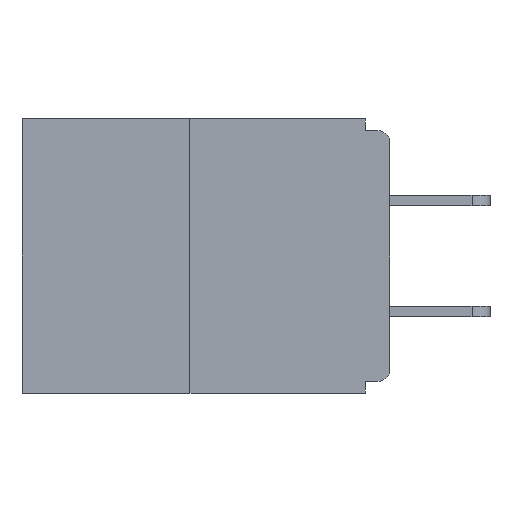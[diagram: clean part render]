
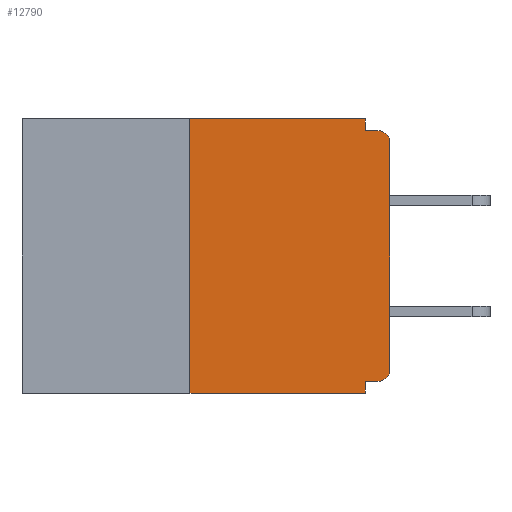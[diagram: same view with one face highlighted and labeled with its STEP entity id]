
A CAD part, left-side view. The second image highlights one B-rep face of the part: STEP entity #12790.
In plain terms, the highlighted planar face has unit normal (-1, 0, 0).
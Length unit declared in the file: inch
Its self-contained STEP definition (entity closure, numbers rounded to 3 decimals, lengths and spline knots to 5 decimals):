
#54 = VECTOR ( 'NONE', #16670, 39.37008 ) ;
#534 = VECTOR ( 'NONE', #2295, 39.37008 ) ;
#1168 = CARTESIAN_POINT ( 'NONE',  ( 0., 0.031, -0.343 ) ) ;
#1472 = CARTESIAN_POINT ( 'NONE',  ( 0., 0.46, 0. ) ) ;
#1593 = DIRECTION ( 'NONE',  ( 0., 0., -1. ) ) ;
#1607 = ORIENTED_EDGE ( 'NONE', *, *, #25234, .F. ) ;
#1665 = LINE ( 'NONE', #11369, #534 ) ;
#2192 = ORIENTED_EDGE ( 'NONE', *, *, #21940, .F. ) ;
#2295 = DIRECTION ( 'NONE',  ( 0., -1., 0. ) ) ;
#2840 = DIRECTION ( 'NONE',  ( 0., 0., -1. ) ) ;
#3822 = CARTESIAN_POINT ( 'NONE',  ( 0., 0.25, 0. ) ) ;
#4606 = EDGE_CURVE ( 'NONE', #22993, #29356, #28138, .T. ) ;
#4746 = CARTESIAN_POINT ( 'NONE',  ( 0., 0.015, -0.313 ) ) ;
#4749 = VERTEX_POINT ( 'NONE', #10541 ) ;
#4824 = CARTESIAN_POINT ( 'NONE',  ( 0., 0., -0.03 ) ) ;
#4848 = VECTOR ( 'NONE', #27370, 39.37008 ) ;
#4927 = CARTESIAN_POINT ( 'NONE',  ( 0., 0.031, 0. ) ) ;
#5744 = ORIENTED_EDGE ( 'NONE', *, *, #18024, .T. ) ;
#6052 = PLANE ( 'NONE',  #17828 ) ;
#6972 = EDGE_CURVE ( 'NONE', #29356, #10993, #19024, .T. ) ;
#7485 = CARTESIAN_POINT ( 'NONE',  ( 0., 0.25, 0. ) ) ;
#7490 = ORIENTED_EDGE ( 'NONE', *, *, #10183, .T. ) ;
#7492 = CIRCLE ( 'NONE', #15079, 0.015 ) ;
#7912 = VERTEX_POINT ( 'NONE', #4824 ) ;
#7968 = VERTEX_POINT ( 'NONE', #7485 ) ;
#8886 = LINE ( 'NONE', #9235, #4848 ) ;
#8995 = AXIS2_PLACEMENT_3D ( 'NONE', #4746, #16107, #18436 ) ;
#9235 = CARTESIAN_POINT ( 'NONE',  ( 0., 0., 0. ) ) ;
#9342 = CARTESIAN_POINT ( 'NONE',  ( 0., 0.46, -0.343 ) ) ;
#9534 = DIRECTION ( 'NONE',  ( 0., -1., 0. ) ) ;
#10183 = EDGE_CURVE ( 'NONE', #7912, #10993, #7492, .T. ) ;
#10427 = DIRECTION ( 'NONE',  ( 0., -1., 0. ) ) ;
#10441 = LINE ( 'NONE', #9342, #25332 ) ;
#10483 = EDGE_CURVE ( 'NONE', #15209, #23033, #10441, .T. ) ;
#10541 = CARTESIAN_POINT ( 'NONE',  ( 0., 0.031, -0.328 ) ) ;
#10993 = VERTEX_POINT ( 'NONE', #16839 ) ;
#11369 = CARTESIAN_POINT ( 'NONE',  ( 0., 0.46, 0. ) ) ;
#11715 = ORIENTED_EDGE ( 'NONE', *, *, #20308, .F. ) ;
#11985 = CARTESIAN_POINT ( 'NONE',  ( 0., 0., -0.015 ) ) ;
#12378 = CARTESIAN_POINT ( 'NONE',  ( 0., 0.25, -0.343 ) ) ;
#12790 = ADVANCED_FACE ( 'NONE', ( #25566 ), #6052, .F. ) ;
#13794 = EDGE_CURVE ( 'NONE', #14344, #4749, #19352, .T. ) ;
#14111 = ORIENTED_EDGE ( 'NONE', *, *, #13794, .F. ) ;
#14344 = VERTEX_POINT ( 'NONE', #16076 ) ;
#15079 = AXIS2_PLACEMENT_3D ( 'NONE', #19094, #26093, #28530 ) ;
#15209 = VERTEX_POINT ( 'NONE', #12378 ) ;
#15305 = EDGE_LOOP ( 'NONE', ( #1607, #2192, #17793, #11715, #14111, #20215, #5744, #7490, #19485, #23784 ) ) ;
#16076 = CARTESIAN_POINT ( 'NONE',  ( 0., 0.015, -0.328 ) ) ;
#16107 = DIRECTION ( 'NONE',  ( -1., 0., 0. ) ) ;
#16670 = DIRECTION ( 'NONE',  ( 0., 0., -1. ) ) ;
#16839 = CARTESIAN_POINT ( 'NONE',  ( 0., 0.015, -0.015 ) ) ;
#16974 = CARTESIAN_POINT ( 'NONE',  ( 0., 0.031, 0. ) ) ;
#17793 = ORIENTED_EDGE ( 'NONE', *, *, #10483, .T. ) ;
#17804 = VERTEX_POINT ( 'NONE', #23931 ) ;
#17828 = AXIS2_PLACEMENT_3D ( 'NONE', #1472, #27124, #1593 ) ;
#18024 = EDGE_CURVE ( 'NONE', #17804, #7912, #8886, .T. ) ;
#18436 = DIRECTION ( 'NONE',  ( 0., 0., -1. ) ) ;
#18606 = VECTOR ( 'NONE', #25016, 39.37008 ) ;
#19024 = LINE ( 'NONE', #11985, #19764 ) ;
#19094 = CARTESIAN_POINT ( 'NONE',  ( 0., 0.015, -0.03 ) ) ;
#19352 = LINE ( 'NONE', #22488, #18606 ) ;
#19485 = ORIENTED_EDGE ( 'NONE', *, *, #6972, .F. ) ;
#19764 = VECTOR ( 'NONE', #9534, 39.37008 ) ;
#20215 = ORIENTED_EDGE ( 'NONE', *, *, #20249, .T. ) ;
#20249 = EDGE_CURVE ( 'NONE', #14344, #17804, #22979, .T. ) ;
#20308 = EDGE_CURVE ( 'NONE', #4749, #23033, #28054, .T. ) ;
#20576 = CARTESIAN_POINT ( 'NONE',  ( 0., 0.031, -0.015 ) ) ;
#21549 = VECTOR ( 'NONE', #2840, 39.37008 ) ;
#21812 = VECTOR ( 'NONE', #29374, 39.37008 ) ;
#21940 = EDGE_CURVE ( 'NONE', #15209, #7968, #27977, .T. ) ;
#22488 = CARTESIAN_POINT ( 'NONE',  ( 0., 0., -0.328 ) ) ;
#22979 = CIRCLE ( 'NONE', #8995, 0.015 ) ;
#22993 = VERTEX_POINT ( 'NONE', #16974 ) ;
#23033 = VERTEX_POINT ( 'NONE', #1168 ) ;
#23784 = ORIENTED_EDGE ( 'NONE', *, *, #4606, .F. ) ;
#23931 = CARTESIAN_POINT ( 'NONE',  ( 0., 0., -0.313 ) ) ;
#25016 = DIRECTION ( 'NONE',  ( 0., 1., 0. ) ) ;
#25234 = EDGE_CURVE ( 'NONE', #7968, #22993, #1665, .T. ) ;
#25332 = VECTOR ( 'NONE', #10427, 39.37008 ) ;
#25566 = FACE_OUTER_BOUND ( 'NONE', #15305, .T. ) ;
#26093 = DIRECTION ( 'NONE',  ( -1., 0., 0. ) ) ;
#27124 = DIRECTION ( 'NONE',  ( 1., 0., 0. ) ) ;
#27370 = DIRECTION ( 'NONE',  ( 0., 0., 1. ) ) ;
#27977 = LINE ( 'NONE', #3822, #21812 ) ;
#28054 = LINE ( 'NONE', #28372, #21549 ) ;
#28138 = LINE ( 'NONE', #4927, #54 ) ;
#28372 = CARTESIAN_POINT ( 'NONE',  ( 0., 0.031, -0.343 ) ) ;
#28530 = DIRECTION ( 'NONE',  ( 0., 0., -1. ) ) ;
#29356 = VERTEX_POINT ( 'NONE', #20576 ) ;
#29374 = DIRECTION ( 'NONE',  ( 0., 0., 1. ) ) ;
